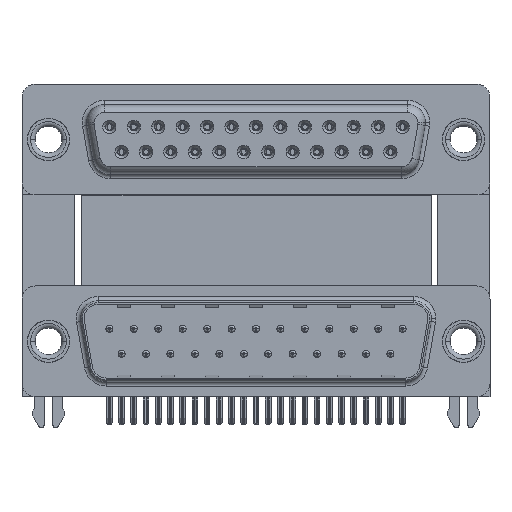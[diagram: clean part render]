
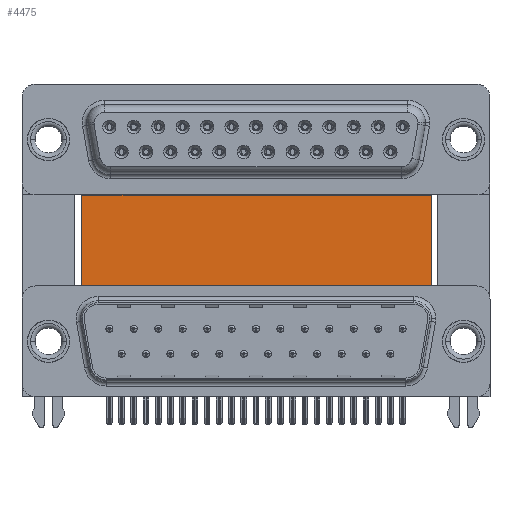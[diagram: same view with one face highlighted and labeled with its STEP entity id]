
A CAD part, top view. The second image highlights one B-rep face of the part: STEP entity #4475.
In plain terms, the highlighted planar face has unit normal (0, 0, 1).
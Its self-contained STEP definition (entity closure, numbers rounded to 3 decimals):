
#776 = DIRECTION ( 'NONE',  ( 1., 0., 0. ) ) ;
#4475 = ADVANCED_FACE ( 'NONE', ( #20223 ), #50897, .F. ) ;
#5506 = ORIENTED_EDGE ( 'NONE', *, *, #7065, .T. ) ;
#5940 = EDGE_CURVE ( 'NONE', #47814, #33132, #7037, .T. ) ;
#7037 = LINE ( 'NONE', #32951, #47563 ) ;
#7065 = EDGE_CURVE ( 'NONE', #27947, #47814, #10742, .T. ) ;
#10198 = DIRECTION ( 'NONE',  ( 0., -1., 0. ) ) ;
#10742 = LINE ( 'NONE', #28016, #48399 ) ;
#11971 = CARTESIAN_POINT ( 'NONE',  ( 3.79, 16.585, -12. ) ) ;
#13333 = LINE ( 'NONE', #21701, #43477 ) ;
#17734 = LINE ( 'NONE', #38402, #31879 ) ;
#18614 = CARTESIAN_POINT ( 'NONE',  ( 43.43, 16.585, -12. ) ) ;
#20223 = FACE_OUTER_BOUND ( 'NONE', #46302, .T. ) ;
#21701 = CARTESIAN_POINT ( 'NONE',  ( 3.79, 16.585, -12. ) ) ;
#25253 = CARTESIAN_POINT ( 'NONE',  ( 3.79, 16.585, -12. ) ) ;
#26001 = ORIENTED_EDGE ( 'NONE', *, *, #52142, .F. ) ;
#26233 = CARTESIAN_POINT ( 'NONE',  ( 43.43, -3.735, -12. ) ) ;
#27036 = ORIENTED_EDGE ( 'NONE', *, *, #5940, .T. ) ;
#27947 = VERTEX_POINT ( 'NONE', #11971 ) ;
#28016 = CARTESIAN_POINT ( 'NONE',  ( 3.79, 16.585, -12. ) ) ;
#28263 = VERTEX_POINT ( 'NONE', #18614 ) ;
#31879 = VECTOR ( 'NONE', #38672, 1000. ) ;
#32951 = CARTESIAN_POINT ( 'NONE',  ( 3.79, -3.735, -12. ) ) ;
#33132 = VERTEX_POINT ( 'NONE', #26233 ) ;
#35308 = AXIS2_PLACEMENT_3D ( 'NONE', #25253, #37799, #46164 ) ;
#36870 = DIRECTION ( 'NONE',  ( 1., 0., 0. ) ) ;
#37799 = DIRECTION ( 'NONE',  ( 0., 0., -1. ) ) ;
#38402 = CARTESIAN_POINT ( 'NONE',  ( 43.43, 16.585, -12. ) ) ;
#38672 = DIRECTION ( 'NONE',  ( 0., -1., 0. ) ) ;
#43477 = VECTOR ( 'NONE', #776, 1000. ) ;
#43859 = ORIENTED_EDGE ( 'NONE', *, *, #54128, .F. ) ;
#45404 = CARTESIAN_POINT ( 'NONE',  ( 3.79, -3.735, -12. ) ) ;
#46164 = DIRECTION ( 'NONE',  ( -1., 0., 0. ) ) ;
#46302 = EDGE_LOOP ( 'NONE', ( #27036, #26001, #43859, #5506 ) ) ;
#47563 = VECTOR ( 'NONE', #36870, 1000. ) ;
#47814 = VERTEX_POINT ( 'NONE', #45404 ) ;
#48399 = VECTOR ( 'NONE', #10198, 1000. ) ;
#50897 = PLANE ( 'NONE',  #35308 ) ;
#52142 = EDGE_CURVE ( 'NONE', #28263, #33132, #17734, .T. ) ;
#54128 = EDGE_CURVE ( 'NONE', #27947, #28263, #13333, .T. ) ;
